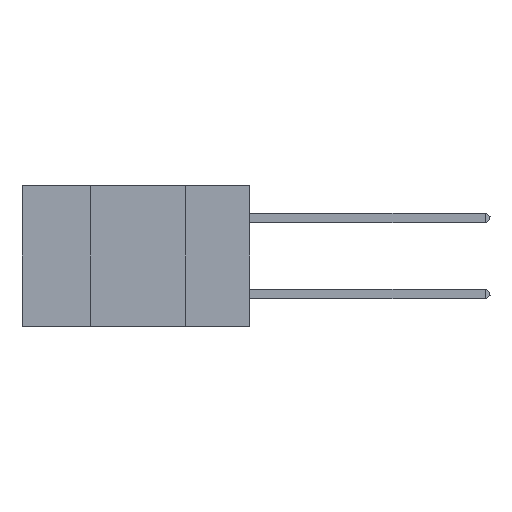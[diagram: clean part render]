
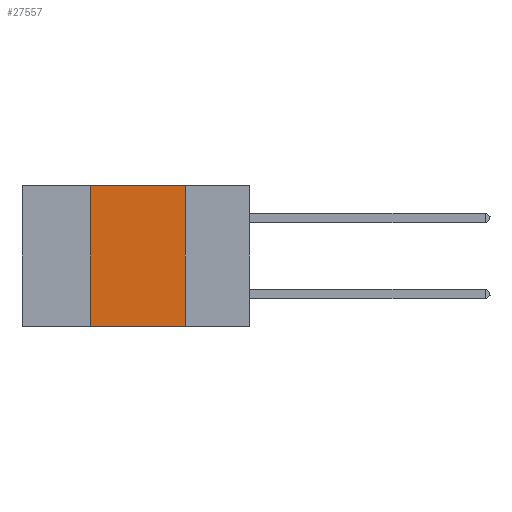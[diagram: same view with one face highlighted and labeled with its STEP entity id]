
A CAD part, left-side view. The second image highlights one B-rep face of the part: STEP entity #27557.
In plain terms, the highlighted planar face has unit normal (-1, 0, 0).
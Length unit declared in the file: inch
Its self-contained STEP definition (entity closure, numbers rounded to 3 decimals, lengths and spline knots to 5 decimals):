
#1048 = DIRECTION ( 'NONE',  ( 0., 0., -1. ) ) ;
#2254 = LINE ( 'NONE', #7690, #15909 ) ;
#2524 = VECTOR ( 'NONE', #35055, 39.37008 ) ;
#4213 = VERTEX_POINT ( 'NONE', #13552 ) ;
#4987 = CARTESIAN_POINT ( 'NONE',  ( 0., 0.17, 0. ) ) ;
#5468 = DIRECTION ( 'NONE',  ( 0., 0., -1. ) ) ;
#6269 = ORIENTED_EDGE ( 'NONE', *, *, #29980, .F. ) ;
#7690 = CARTESIAN_POINT ( 'NONE',  ( 0., 0.6, -0.37 ) ) ;
#8258 = CARTESIAN_POINT ( 'NONE',  ( 0., 0.6, 0. ) ) ;
#8988 = VERTEX_POINT ( 'NONE', #4987 ) ;
#9755 = CARTESIAN_POINT ( 'NONE',  ( 0., 0.42, 0. ) ) ;
#11117 = FACE_OUTER_BOUND ( 'NONE', #31904, .T. ) ;
#11582 = ORIENTED_EDGE ( 'NONE', *, *, #14688, .T. ) ;
#12252 = CARTESIAN_POINT ( 'NONE',  ( 0., 0.42, -0.37 ) ) ;
#12576 = LINE ( 'NONE', #33101, #23107 ) ;
#13552 = CARTESIAN_POINT ( 'NONE',  ( 0., 0.17, -0.37 ) ) ;
#14688 = EDGE_CURVE ( 'NONE', #21045, #4213, #2254, .T. ) ;
#15909 = VECTOR ( 'NONE', #36626, 39.37008 ) ;
#17295 = LINE ( 'NONE', #36617, #35512 ) ;
#20951 = EDGE_CURVE ( 'NONE', #21045, #26324, #34416, .T. ) ;
#21045 = VERTEX_POINT ( 'NONE', #12252 ) ;
#22908 = DIRECTION ( 'NONE',  ( 1., 0., 0. ) ) ;
#23107 = VECTOR ( 'NONE', #1048, 39.37008 ) ;
#25733 = EDGE_CURVE ( 'NONE', #8988, #4213, #12576, .T. ) ;
#26324 = VERTEX_POINT ( 'NONE', #9755 ) ;
#26432 = ORIENTED_EDGE ( 'NONE', *, *, #20951, .F. ) ;
#26741 = ORIENTED_EDGE ( 'NONE', *, *, #25733, .F. ) ;
#27557 = ADVANCED_FACE ( 'NONE', ( #11117 ), #31698, .F. ) ;
#29980 = EDGE_CURVE ( 'NONE', #26324, #8988, #17295, .T. ) ;
#31013 = AXIS2_PLACEMENT_3D ( 'NONE', #8258, #22908, #5468 ) ;
#31260 = DIRECTION ( 'NONE',  ( 0., -1., 0. ) ) ;
#31698 = PLANE ( 'NONE',  #31013 ) ;
#31904 = EDGE_LOOP ( 'NONE', ( #26741, #6269, #26432, #11582 ) ) ;
#32386 = CARTESIAN_POINT ( 'NONE',  ( 0., 0.42, 0. ) ) ;
#33101 = CARTESIAN_POINT ( 'NONE',  ( 0., 0.17, 0. ) ) ;
#34416 = LINE ( 'NONE', #32386, #2524 ) ;
#35055 = DIRECTION ( 'NONE',  ( 0., 0., 1. ) ) ;
#35512 = VECTOR ( 'NONE', #31260, 39.37008 ) ;
#36617 = CARTESIAN_POINT ( 'NONE',  ( 0., 0.6, 0. ) ) ;
#36626 = DIRECTION ( 'NONE',  ( 0., -1., 0. ) ) ;
